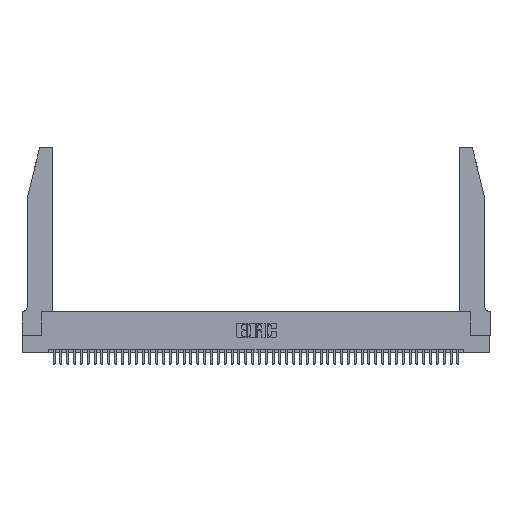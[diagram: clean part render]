
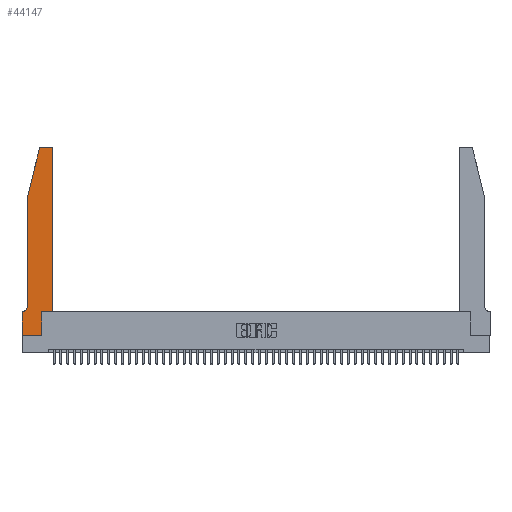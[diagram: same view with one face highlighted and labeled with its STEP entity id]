
A CAD part, top view. The second image highlights one B-rep face of the part: STEP entity #44147.
In plain terms, the highlighted planar face has unit normal (0, 0, 1).
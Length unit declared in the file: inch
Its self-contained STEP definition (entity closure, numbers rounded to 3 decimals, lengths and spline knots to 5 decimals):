
#489 = LINE ( 'NONE', #20494, #21406 ) ;
#815 = VECTOR ( 'NONE', #3083, 39.37008 ) ;
#1233 = EDGE_CURVE ( 'NONE', #19898, #22791, #34081, .T. ) ;
#1328 = EDGE_CURVE ( 'NONE', #22791, #36886, #4750, .T. ) ;
#1558 = DIRECTION ( 'NONE',  ( 1., 0., 0. ) ) ;
#1732 = DIRECTION ( 'NONE',  ( -1., 0., 0. ) ) ;
#1904 = DIRECTION ( 'NONE',  ( 0., 0., 1. ) ) ;
#2519 = LINE ( 'NONE', #22572, #13813 ) ;
#2927 = CARTESIAN_POINT ( 'NONE',  ( 0., 0., 0.37 ) ) ;
#3083 = DIRECTION ( 'NONE',  ( -0.239, -0.971, 0. ) ) ;
#3477 = DIRECTION ( 'NONE',  ( 0., 0., -1. ) ) ;
#3980 = LINE ( 'NONE', #8839, #25548 ) ;
#4750 = LINE ( 'NONE', #9366, #31667 ) ;
#5150 = CARTESIAN_POINT ( 'NONE',  ( 0., 0.35, 0.37 ) ) ;
#5546 = VERTEX_POINT ( 'NONE', #9149 ) ;
#5958 = EDGE_CURVE ( 'NONE', #5546, #19898, #2519, .T. ) ;
#7056 = CARTESIAN_POINT ( 'NONE',  ( 0.0755, 2., 0.37 ) ) ;
#7500 = ORIENTED_EDGE ( 'NONE', *, *, #1328, .T. ) ;
#7531 = FACE_OUTER_BOUND ( 'NONE', #45180, .T. ) ;
#7565 = ORIENTED_EDGE ( 'NONE', *, *, #5958, .T. ) ;
#7609 = VECTOR ( 'NONE', #42959, 39.37008 ) ;
#8839 = CARTESIAN_POINT ( 'NONE',  ( 0., 0., 0.37 ) ) ;
#9149 = CARTESIAN_POINT ( 'NONE',  ( 0.4505, 0.35, 0.37 ) ) ;
#9366 = CARTESIAN_POINT ( 'NONE',  ( 0.2605, 2.75, 0.37 ) ) ;
#9842 = ORIENTED_EDGE ( 'NONE', *, *, #13837, .T. ) ;
#10560 = DIRECTION ( 'NONE',  ( 0., -1., 0. ) ) ;
#11810 = ORIENTED_EDGE ( 'NONE', *, *, #31658, .T. ) ;
#11909 = EDGE_CURVE ( 'NONE', #49526, #17252, #17930, .T. ) ;
#12257 = CARTESIAN_POINT ( 'NONE',  ( 0.0755, 2., 0.37 ) ) ;
#13039 = VECTOR ( 'NONE', #26510, 39.37008 ) ;
#13813 = VECTOR ( 'NONE', #23081, 39.37008 ) ;
#13837 = EDGE_CURVE ( 'NONE', #15368, #49526, #49539, .T. ) ;
#14243 = LINE ( 'NONE', #49382, #13039 ) ;
#14270 = DIRECTION ( 'NONE',  ( 1., 0., 0. ) ) ;
#15123 = VERTEX_POINT ( 'NONE', #5150 ) ;
#15167 = CARTESIAN_POINT ( 'NONE',  ( 0.284, 2.72, 0.37 ) ) ;
#15368 = VERTEX_POINT ( 'NONE', #25599 ) ;
#15644 = ORIENTED_EDGE ( 'NONE', *, *, #34467, .T. ) ;
#16410 = DIRECTION ( 'NONE',  ( 1., 0., 0. ) ) ;
#16629 = VERTEX_POINT ( 'NONE', #25198 ) ;
#16742 = EDGE_CURVE ( 'NONE', #17252, #15123, #30593, .T. ) ;
#17252 = VERTEX_POINT ( 'NONE', #43705 ) ;
#17930 = CIRCLE ( 'NONE', #32694, 0.07 ) ;
#18271 = DIRECTION ( 'NONE',  ( -1., 0., 0. ) ) ;
#18572 = EDGE_CURVE ( 'NONE', #15123, #42315, #40595, .T. ) ;
#18948 = VERTEX_POINT ( 'NONE', #31975 ) ;
#19898 = VERTEX_POINT ( 'NONE', #26459 ) ;
#20494 = CARTESIAN_POINT ( 'NONE',  ( 0.2865, 0.35, 0.37 ) ) ;
#21406 = VECTOR ( 'NONE', #28568, 39.37008 ) ;
#21744 = ORIENTED_EDGE ( 'NONE', *, *, #25685, .T. ) ;
#22572 = CARTESIAN_POINT ( 'NONE',  ( 0.4505, 0.35, 0.37 ) ) ;
#22736 = DIRECTION ( 'NONE',  ( 0., 0., 1. ) ) ;
#22791 = VERTEX_POINT ( 'NONE', #33799 ) ;
#23081 = DIRECTION ( 'NONE',  ( 0., 1., 0. ) ) ;
#24168 = LINE ( 'NONE', #7056, #815 ) ;
#24305 = EDGE_CURVE ( 'NONE', #16629, #5546, #14243, .T. ) ;
#25198 = CARTESIAN_POINT ( 'NONE',  ( 0.2865, 0.35, 0.37 ) ) ;
#25547 = CARTESIAN_POINT ( 'NONE',  ( 0., 0.35, 0.37 ) ) ;
#25548 = VECTOR ( 'NONE', #16410, 39.37008 ) ;
#25599 = CARTESIAN_POINT ( 'NONE',  ( 0.0755, 2., 0.37 ) ) ;
#25685 = EDGE_CURVE ( 'NONE', #42315, #18948, #3980, .T. ) ;
#26200 = VERTEX_POINT ( 'NONE', #42528 ) ;
#26459 = CARTESIAN_POINT ( 'NONE',  ( 0.4505, 2.72, 0.37 ) ) ;
#26510 = DIRECTION ( 'NONE',  ( 1., 0., 0. ) ) ;
#26826 = ORIENTED_EDGE ( 'NONE', *, *, #16742, .T. ) ;
#28568 = DIRECTION ( 'NONE',  ( 0., 1., 0. ) ) ;
#30395 = VECTOR ( 'NONE', #10560, 39.37008 ) ;
#30520 = CARTESIAN_POINT ( 'NONE',  ( 0.0755, 0.42, 0.37 ) ) ;
#30593 = LINE ( 'NONE', #33708, #31772 ) ;
#31658 = EDGE_CURVE ( 'NONE', #26200, #15368, #24168, .T. ) ;
#31667 = VECTOR ( 'NONE', #1732, 39.37008 ) ;
#31772 = VECTOR ( 'NONE', #18271, 39.37008 ) ;
#31975 = CARTESIAN_POINT ( 'NONE',  ( 0.2865, 0., 0.37 ) ) ;
#32694 = AXIS2_PLACEMENT_3D ( 'NONE', #49303, #3477, #34096 ) ;
#33013 = CARTESIAN_POINT ( 'NONE',  ( 0.284, 2.75, 0.37 ) ) ;
#33566 = PLANE ( 'NONE',  #47978 ) ;
#33708 = CARTESIAN_POINT ( 'NONE',  ( 0.0755, 0.35, 0.37 ) ) ;
#33799 = CARTESIAN_POINT ( 'NONE',  ( 0.4205, 2.75, 0.37 ) ) ;
#34081 = CIRCLE ( 'NONE', #43345, 0.03 ) ;
#34096 = DIRECTION ( 'NONE',  ( -1., 0., 0. ) ) ;
#34440 = DIRECTION ( 'NONE',  ( 1., 0., 0. ) ) ;
#34467 = EDGE_CURVE ( 'NONE', #36886, #26200, #37068, .T. ) ;
#34791 = EDGE_CURVE ( 'NONE', #18948, #16629, #489, .T. ) ;
#35566 = ORIENTED_EDGE ( 'NONE', *, *, #1233, .T. ) ;
#36886 = VERTEX_POINT ( 'NONE', #33013 ) ;
#37068 = CIRCLE ( 'NONE', #38997, 0.03 ) ;
#37282 = DIRECTION ( 'NONE',  ( 0., 0., 1. ) ) ;
#38997 = AXIS2_PLACEMENT_3D ( 'NONE', #15167, #22736, #34440 ) ;
#40255 = CARTESIAN_POINT ( 'NONE',  ( 0.4205, 2.72, 0.37 ) ) ;
#40595 = LINE ( 'NONE', #2927, #30395 ) ;
#41689 = ORIENTED_EDGE ( 'NONE', *, *, #24305, .T. ) ;
#42315 = VERTEX_POINT ( 'NONE', #48596 ) ;
#42528 = CARTESIAN_POINT ( 'NONE',  ( 0.25487, 2.72718, 0.37 ) ) ;
#42959 = DIRECTION ( 'NONE',  ( 0., -1., 0. ) ) ;
#43345 = AXIS2_PLACEMENT_3D ( 'NONE', #40255, #1904, #1558 ) ;
#43705 = CARTESIAN_POINT ( 'NONE',  ( 0.0055, 0.35, 0.37 ) ) ;
#44147 = ADVANCED_FACE ( 'NONE', ( #7531 ), #33566, .T. ) ;
#45180 = EDGE_LOOP ( 'NONE', ( #7500, #15644, #11810, #9842, #46208, #26826, #47398, #21744, #45309, #41689, #7565, #35566 ) ) ;
#45309 = ORIENTED_EDGE ( 'NONE', *, *, #34791, .T. ) ;
#46208 = ORIENTED_EDGE ( 'NONE', *, *, #11909, .T. ) ;
#47398 = ORIENTED_EDGE ( 'NONE', *, *, #18572, .T. ) ;
#47978 = AXIS2_PLACEMENT_3D ( 'NONE', #25547, #37282, #14270 ) ;
#48596 = CARTESIAN_POINT ( 'NONE',  ( 0., 0., 0.37 ) ) ;
#49303 = CARTESIAN_POINT ( 'NONE',  ( 0.0055, 0.42, 0.37 ) ) ;
#49382 = CARTESIAN_POINT ( 'NONE',  ( 0.4505, 0.35, 0.37 ) ) ;
#49526 = VERTEX_POINT ( 'NONE', #30520 ) ;
#49539 = LINE ( 'NONE', #12257, #7609 ) ;
